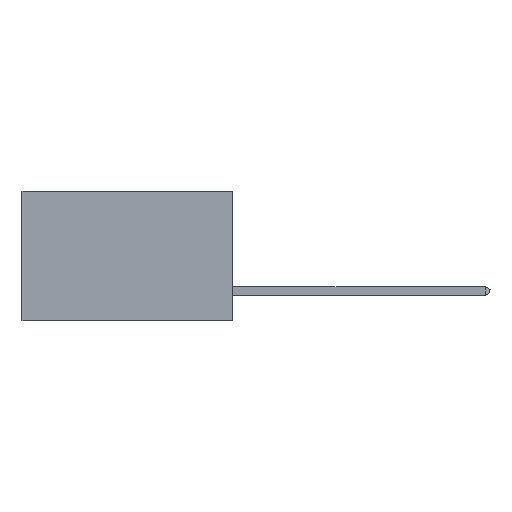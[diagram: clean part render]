
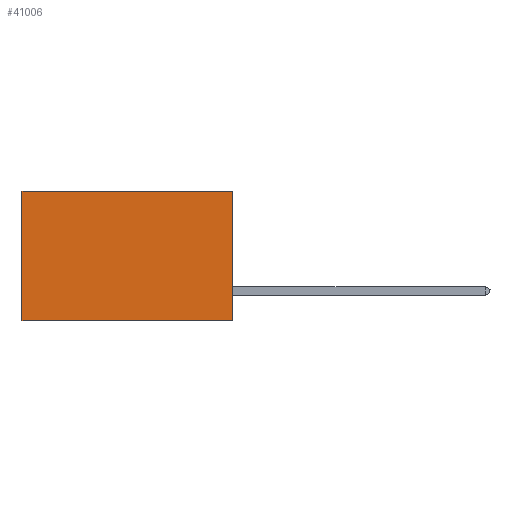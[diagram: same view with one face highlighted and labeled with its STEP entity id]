
A CAD part, left-side view. The second image highlights one B-rep face of the part: STEP entity #41006.
In plain terms, the highlighted planar face has unit normal (-1, 0, 0).
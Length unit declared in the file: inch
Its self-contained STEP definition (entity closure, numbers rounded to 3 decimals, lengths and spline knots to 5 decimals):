
#478 = AXIS2_PLACEMENT_3D ( 'NONE', #4131, #22224, #18492 ) ;
#555 = VECTOR ( 'NONE', #10287, 39.37008 ) ;
#3105 = LINE ( 'NONE', #45277, #26114 ) ;
#3360 = VECTOR ( 'NONE', #8863, 39.37008 ) ;
#4131 = CARTESIAN_POINT ( 'NONE',  ( 0.2875, 0., 0. ) ) ;
#4235 = EDGE_CURVE ( 'NONE', #13369, #15557, #40124, .T. ) ;
#8863 = DIRECTION ( 'NONE',  ( 0., 0., -1. ) ) ;
#10287 = DIRECTION ( 'NONE',  ( 0., 1., 0. ) ) ;
#12390 = CARTESIAN_POINT ( 'NONE',  ( 0.2875, 0., -0.37 ) ) ;
#13013 = ORIENTED_EDGE ( 'NONE', *, *, #34696, .F. ) ;
#13096 = FACE_OUTER_BOUND ( 'NONE', #34039, .T. ) ;
#13314 = VERTEX_POINT ( 'NONE', #16511 ) ;
#13369 = VERTEX_POINT ( 'NONE', #18804 ) ;
#14178 = ORIENTED_EDGE ( 'NONE', *, *, #31932, .T. ) ;
#15557 = VERTEX_POINT ( 'NONE', #33786 ) ;
#16511 = CARTESIAN_POINT ( 'NONE',  ( 0.2875, 0., 0. ) ) ;
#18492 = DIRECTION ( 'NONE',  ( 0., 0., -1. ) ) ;
#18804 = CARTESIAN_POINT ( 'NONE',  ( 0.2875, 0., -0.37 ) ) ;
#21569 = CARTESIAN_POINT ( 'NONE',  ( 0.2875, 0., 0. ) ) ;
#21905 = ORIENTED_EDGE ( 'NONE', *, *, #36053, .T. ) ;
#22224 = DIRECTION ( 'NONE',  ( 1., 0., 0. ) ) ;
#23131 = LINE ( 'NONE', #21569, #555 ) ;
#25021 = CARTESIAN_POINT ( 'NONE',  ( 0.2875, 0.6, 0. ) ) ;
#26114 = VECTOR ( 'NONE', #38085, 39.37008 ) ;
#30573 = VECTOR ( 'NONE', #41236, 39.37008 ) ;
#31932 = EDGE_CURVE ( 'NONE', #43589, #15557, #45565, .T. ) ;
#33786 = CARTESIAN_POINT ( 'NONE',  ( 0.2875, 0.6, -0.37 ) ) ;
#34039 = EDGE_LOOP ( 'NONE', ( #14178, #36691, #13013, #21905 ) ) ;
#34696 = EDGE_CURVE ( 'NONE', #13314, #13369, #3105, .T. ) ;
#36053 = EDGE_CURVE ( 'NONE', #13314, #43589, #23131, .T. ) ;
#36691 = ORIENTED_EDGE ( 'NONE', *, *, #4235, .F. ) ;
#38085 = DIRECTION ( 'NONE',  ( 0., 0., -1. ) ) ;
#40067 = PLANE ( 'NONE',  #478 ) ;
#40124 = LINE ( 'NONE', #12390, #30573 ) ;
#41006 = ADVANCED_FACE ( 'NONE', ( #13096 ), #40067, .F. ) ;
#41152 = CARTESIAN_POINT ( 'NONE',  ( 0.2875, 0.6, 0. ) ) ;
#41236 = DIRECTION ( 'NONE',  ( 0., 1., 0. ) ) ;
#43589 = VERTEX_POINT ( 'NONE', #25021 ) ;
#45277 = CARTESIAN_POINT ( 'NONE',  ( 0.2875, 0., 0. ) ) ;
#45565 = LINE ( 'NONE', #41152, #3360 ) ;
